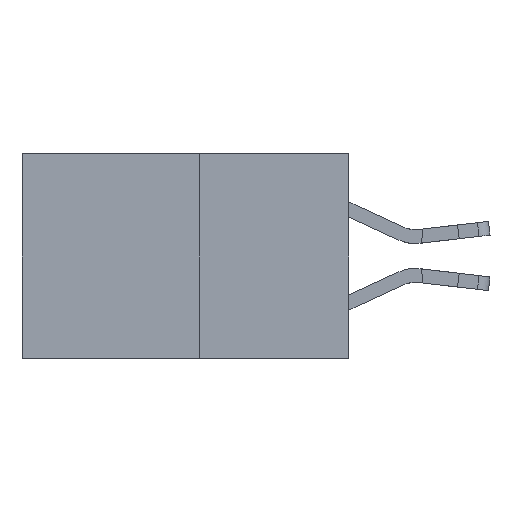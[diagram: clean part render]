
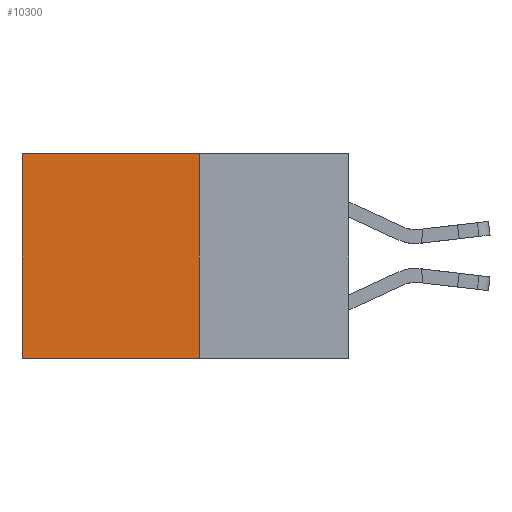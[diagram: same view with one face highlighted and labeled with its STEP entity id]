
A CAD part, left-side view. The second image highlights one B-rep face of the part: STEP entity #10300.
In plain terms, the highlighted planar face has unit normal (-1, 0, 0).
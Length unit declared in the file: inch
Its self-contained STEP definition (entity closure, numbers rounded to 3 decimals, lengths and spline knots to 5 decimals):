
#680 = ORIENTED_EDGE ( 'NONE', *, *, #10012, .T. ) ;
#1376 = CARTESIAN_POINT ( 'NONE',  ( 0.277, 0.27, -0.37 ) ) ;
#1739 = DIRECTION ( 'NONE',  ( 1., 0., 0. ) ) ;
#2650 = CARTESIAN_POINT ( 'NONE',  ( 0.277, 0.27, -0.37 ) ) ;
#4538 = VECTOR ( 'NONE', #7844, 39.37008 ) ;
#5058 = CARTESIAN_POINT ( 'NONE',  ( 0.277, 0.27, -0.37 ) ) ;
#6084 = VECTOR ( 'NONE', #11557, 39.37008 ) ;
#6214 = EDGE_CURVE ( 'NONE', #18162, #20533, #16732, .T. ) ;
#6652 = LINE ( 'NONE', #18690, #6084 ) ;
#7231 = EDGE_LOOP ( 'NONE', ( #680, #8154, #19215, #10547 ) ) ;
#7844 = DIRECTION ( 'NONE',  ( 0., 1., 0. ) ) ;
#8154 = ORIENTED_EDGE ( 'NONE', *, *, #13529, .F. ) ;
#8367 = VECTOR ( 'NONE', #8783, 39.37008 ) ;
#8783 = DIRECTION ( 'NONE',  ( 0., 0., -1. ) ) ;
#9256 = AXIS2_PLACEMENT_3D ( 'NONE', #5058, #1739, #14444 ) ;
#10012 = EDGE_CURVE ( 'NONE', #20533, #19411, #6652, .T. ) ;
#10300 = ADVANCED_FACE ( 'NONE', ( #15701 ), #12657, .F. ) ;
#10547 = ORIENTED_EDGE ( 'NONE', *, *, #6214, .T. ) ;
#10648 = CARTESIAN_POINT ( 'NONE',  ( 0.277, 0.27, 0. ) ) ;
#11288 = CARTESIAN_POINT ( 'NONE',  ( 0.277, 0.59, -0.37 ) ) ;
#11557 = DIRECTION ( 'NONE',  ( 0., 0., -1. ) ) ;
#12490 = CARTESIAN_POINT ( 'NONE',  ( 0.277, 0.27, 0. ) ) ;
#12549 = VECTOR ( 'NONE', #17763, 39.37008 ) ;
#12657 = PLANE ( 'NONE',  #9256 ) ;
#13529 = EDGE_CURVE ( 'NONE', #14849, #19411, #18945, .T. ) ;
#14444 = DIRECTION ( 'NONE',  ( 0., 0., -1. ) ) ;
#14849 = VERTEX_POINT ( 'NONE', #2650 ) ;
#15701 = FACE_OUTER_BOUND ( 'NONE', #7231, .T. ) ;
#16106 = CARTESIAN_POINT ( 'NONE',  ( 0.277, 0.59, 0. ) ) ;
#16732 = LINE ( 'NONE', #12490, #12549 ) ;
#17763 = DIRECTION ( 'NONE',  ( 0., 1., 0. ) ) ;
#17914 = LINE ( 'NONE', #1376, #8367 ) ;
#18142 = EDGE_CURVE ( 'NONE', #18162, #14849, #17914, .T. ) ;
#18162 = VERTEX_POINT ( 'NONE', #10648 ) ;
#18668 = CARTESIAN_POINT ( 'NONE',  ( 0.277, 0.27, -0.37 ) ) ;
#18690 = CARTESIAN_POINT ( 'NONE',  ( 0.277, 0.59, -0.37 ) ) ;
#18945 = LINE ( 'NONE', #18668, #4538 ) ;
#19215 = ORIENTED_EDGE ( 'NONE', *, *, #18142, .F. ) ;
#19411 = VERTEX_POINT ( 'NONE', #11288 ) ;
#20533 = VERTEX_POINT ( 'NONE', #16106 ) ;
